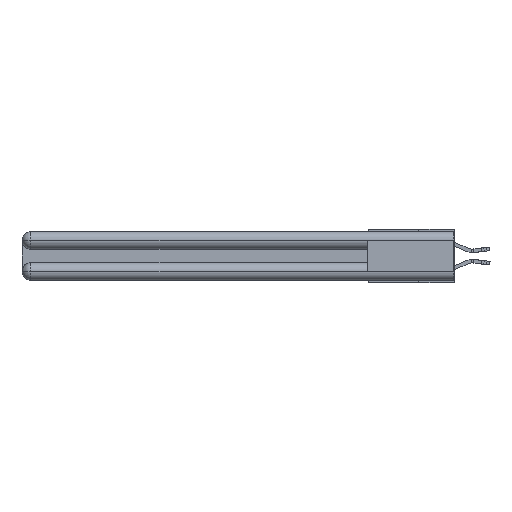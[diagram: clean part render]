
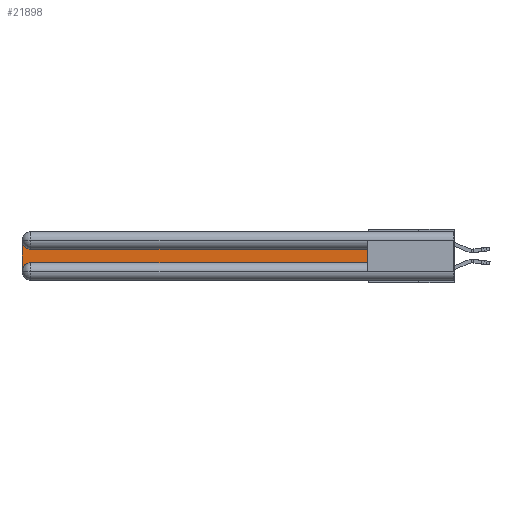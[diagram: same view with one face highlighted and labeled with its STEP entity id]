
A CAD part, left-side view. The second image highlights one B-rep face of the part: STEP entity #21898.
In plain terms, the highlighted planar face has unit normal (-1, 0, 0).
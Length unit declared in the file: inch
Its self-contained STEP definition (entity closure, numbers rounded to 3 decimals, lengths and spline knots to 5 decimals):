
#475 = VERTEX_POINT ( 'NONE', #7104 ) ;
#1595 = EDGE_CURVE ( 'NONE', #475, #25998, #14024, .T. ) ;
#1852 = EDGE_CURVE ( 'NONE', #9963, #9495, #29082, .T. ) ;
#1898 = DIRECTION ( 'NONE',  ( 0., -1., 0. ) ) ;
#2660 = DIRECTION ( 'NONE',  ( 0., 0., -1. ) ) ;
#2963 = ORIENTED_EDGE ( 'NONE', *, *, #13483, .T. ) ;
#3764 = LINE ( 'NONE', #3800, #22009 ) ;
#3800 = CARTESIAN_POINT ( 'NONE',  ( 0.075, 3., -0.2175 ) ) ;
#3872 = CARTESIAN_POINT ( 'NONE',  ( 0.075, 2.94, -0.2775 ) ) ;
#6287 = ORIENTED_EDGE ( 'NONE', *, *, #1595, .T. ) ;
#6382 = CARTESIAN_POINT ( 'NONE',  ( 0.075, 3., -0.0625 ) ) ;
#6501 = ORIENTED_EDGE ( 'NONE', *, *, #13650, .T. ) ;
#6514 = AXIS2_PLACEMENT_3D ( 'NONE', #3872, #10667, #15239 ) ;
#7104 = CARTESIAN_POINT ( 'NONE',  ( 0.075, 0.6, -0.2175 ) ) ;
#9495 = VERTEX_POINT ( 'NONE', #21956 ) ;
#9787 = VERTEX_POINT ( 'NONE', #15080 ) ;
#9963 = VERTEX_POINT ( 'NONE', #21919 ) ;
#10667 = DIRECTION ( 'NONE',  ( 1., 0., 0. ) ) ;
#10809 = PLANE ( 'NONE',  #15524 ) ;
#10877 = LINE ( 'NONE', #26501, #15760 ) ;
#11132 = CIRCLE ( 'NONE', #16041, 0.06 ) ;
#11898 = EDGE_CURVE ( 'NONE', #9787, #12577, #11132, .T. ) ;
#12412 = ORIENTED_EDGE ( 'NONE', *, *, #17558, .T. ) ;
#12577 = VERTEX_POINT ( 'NONE', #6382 ) ;
#13200 = CARTESIAN_POINT ( 'NONE',  ( 0.075, 0.6, -0.1225 ) ) ;
#13483 = EDGE_CURVE ( 'NONE', #12577, #9963, #3764, .T. ) ;
#13650 = EDGE_CURVE ( 'NONE', #9495, #475, #10877, .T. ) ;
#13946 = FACE_OUTER_BOUND ( 'NONE', #27760, .T. ) ;
#14024 = LINE ( 'NONE', #20549, #26257 ) ;
#14651 = ORIENTED_EDGE ( 'NONE', *, *, #11898, .T. ) ;
#15080 = CARTESIAN_POINT ( 'NONE',  ( 0.075, 2.94, -0.1225 ) ) ;
#15239 = DIRECTION ( 'NONE',  ( 0., 0., -1. ) ) ;
#15524 = AXIS2_PLACEMENT_3D ( 'NONE', #28900, #26420, #28703 ) ;
#15760 = VECTOR ( 'NONE', #1898, 39.37008 ) ;
#15961 = ORIENTED_EDGE ( 'NONE', *, *, #1852, .T. ) ;
#16041 = AXIS2_PLACEMENT_3D ( 'NONE', #27493, #16405, #2660 ) ;
#16405 = DIRECTION ( 'NONE',  ( 1., 0., 0. ) ) ;
#16596 = LINE ( 'NONE', #13200, #25352 ) ;
#17558 = EDGE_CURVE ( 'NONE', #25998, #9787, #16596, .T. ) ;
#18301 = DIRECTION ( 'NONE',  ( 0., 0., 1. ) ) ;
#19179 = CARTESIAN_POINT ( 'NONE',  ( 0.075, 0.6, -0.1225 ) ) ;
#20549 = CARTESIAN_POINT ( 'NONE',  ( 0.075, 0.6, -0.2175 ) ) ;
#21898 = ADVANCED_FACE ( 'NONE', ( #13946 ), #10809, .F. ) ;
#21919 = CARTESIAN_POINT ( 'NONE',  ( 0.075, 3., -0.2775 ) ) ;
#21956 = CARTESIAN_POINT ( 'NONE',  ( 0.075, 2.94, -0.2175 ) ) ;
#22009 = VECTOR ( 'NONE', #26213, 39.37008 ) ;
#25352 = VECTOR ( 'NONE', #27021, 39.37008 ) ;
#25998 = VERTEX_POINT ( 'NONE', #19179 ) ;
#26213 = DIRECTION ( 'NONE',  ( 0., 0., -1. ) ) ;
#26257 = VECTOR ( 'NONE', #18301, 39.37008 ) ;
#26420 = DIRECTION ( 'NONE',  ( 1., 0., 0. ) ) ;
#26501 = CARTESIAN_POINT ( 'NONE',  ( 0.075, 0.6, -0.2175 ) ) ;
#27021 = DIRECTION ( 'NONE',  ( 0., 1., 0. ) ) ;
#27493 = CARTESIAN_POINT ( 'NONE',  ( 0.075, 2.94, -0.0625 ) ) ;
#27760 = EDGE_LOOP ( 'NONE', ( #12412, #14651, #2963, #15961, #6501, #6287 ) ) ;
#28703 = DIRECTION ( 'NONE',  ( 0., 0., -1. ) ) ;
#28900 = CARTESIAN_POINT ( 'NONE',  ( 0.075, 3., -0.1225 ) ) ;
#29082 = CIRCLE ( 'NONE', #6514, 0.06 ) ;
